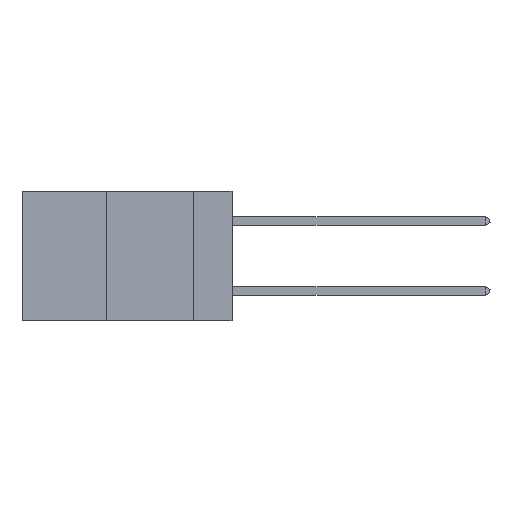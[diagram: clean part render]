
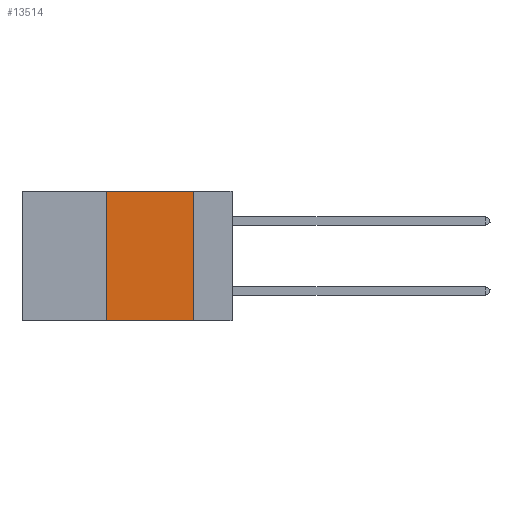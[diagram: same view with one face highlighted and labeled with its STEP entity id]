
A CAD part, left-side view. The second image highlights one B-rep face of the part: STEP entity #13514.
In plain terms, the highlighted planar face has unit normal (-1, 0, 0).
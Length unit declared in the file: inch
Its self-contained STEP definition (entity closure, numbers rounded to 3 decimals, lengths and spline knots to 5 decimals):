
#172 = CARTESIAN_POINT ( 'NONE',  ( 0., 0.36, -0.37 ) ) ;
#1266 = CARTESIAN_POINT ( 'NONE',  ( 0., 0.6, 0. ) ) ;
#1369 = VERTEX_POINT ( 'NONE', #4684 ) ;
#2000 = EDGE_CURVE ( 'NONE', #2286, #11051, #9126, .T. ) ;
#2286 = VERTEX_POINT ( 'NONE', #172 ) ;
#2306 = VECTOR ( 'NONE', #12378, 39.37008 ) ;
#2427 = VECTOR ( 'NONE', #10727, 39.37008 ) ;
#2668 = DIRECTION ( 'NONE',  ( 1., 0., 0. ) ) ;
#4684 = CARTESIAN_POINT ( 'NONE',  ( 0., 0.11, -0.37 ) ) ;
#4837 = CARTESIAN_POINT ( 'NONE',  ( 0., 0.6, -0.37 ) ) ;
#5936 = ORIENTED_EDGE ( 'NONE', *, *, #14559, .F. ) ;
#5954 = ORIENTED_EDGE ( 'NONE', *, *, #7444, .F. ) ;
#6020 = ORIENTED_EDGE ( 'NONE', *, *, #15045, .T. ) ;
#6461 = AXIS2_PLACEMENT_3D ( 'NONE', #1266, #2668, #11637 ) ;
#6551 = ORIENTED_EDGE ( 'NONE', *, *, #2000, .F. ) ;
#6736 = CARTESIAN_POINT ( 'NONE',  ( 0., 0.36, 0. ) ) ;
#7444 = EDGE_CURVE ( 'NONE', #8517, #1369, #9372, .T. ) ;
#7458 = CARTESIAN_POINT ( 'NONE',  ( 0., 0.36, 0. ) ) ;
#8379 = DIRECTION ( 'NONE',  ( 0., 0., 1. ) ) ;
#8517 = VERTEX_POINT ( 'NONE', #9999 ) ;
#8778 = DIRECTION ( 'NONE',  ( 0., -1., 0. ) ) ;
#9126 = LINE ( 'NONE', #6736, #15003 ) ;
#9172 = PLANE ( 'NONE',  #6461 ) ;
#9252 = LINE ( 'NONE', #4837, #2306 ) ;
#9372 = LINE ( 'NONE', #13184, #2427 ) ;
#9999 = CARTESIAN_POINT ( 'NONE',  ( 0., 0.11, 0. ) ) ;
#10727 = DIRECTION ( 'NONE',  ( 0., 0., -1. ) ) ;
#11051 = VERTEX_POINT ( 'NONE', #7458 ) ;
#11637 = DIRECTION ( 'NONE',  ( 0., 0., -1. ) ) ;
#12378 = DIRECTION ( 'NONE',  ( 0., -1., 0. ) ) ;
#12571 = EDGE_LOOP ( 'NONE', ( #5954, #5936, #6551, #6020 ) ) ;
#12826 = VECTOR ( 'NONE', #8778, 39.37008 ) ;
#13184 = CARTESIAN_POINT ( 'NONE',  ( 0., 0.11, 0. ) ) ;
#13194 = LINE ( 'NONE', #13527, #12826 ) ;
#13514 = ADVANCED_FACE ( 'NONE', ( #13603 ), #9172, .F. ) ;
#13527 = CARTESIAN_POINT ( 'NONE',  ( 0., 0.6, 0. ) ) ;
#13603 = FACE_OUTER_BOUND ( 'NONE', #12571, .T. ) ;
#14559 = EDGE_CURVE ( 'NONE', #11051, #8517, #13194, .T. ) ;
#15003 = VECTOR ( 'NONE', #8379, 39.37008 ) ;
#15045 = EDGE_CURVE ( 'NONE', #2286, #1369, #9252, .T. ) ;
